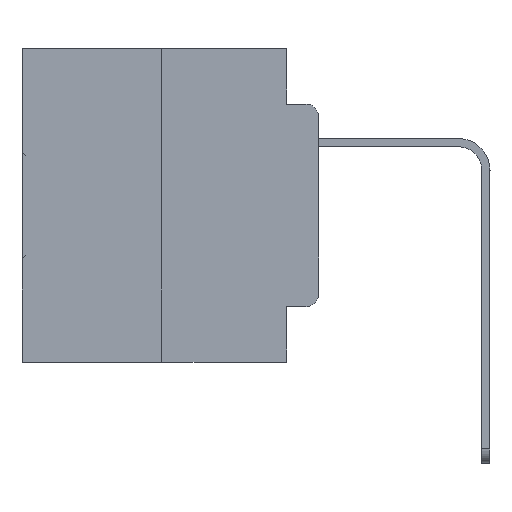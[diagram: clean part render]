
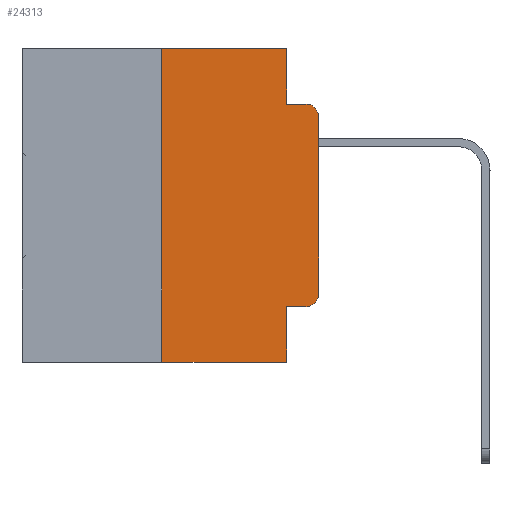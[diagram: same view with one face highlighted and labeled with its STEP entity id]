
A CAD part, left-side view. The second image highlights one B-rep face of the part: STEP entity #24313.
In plain terms, the highlighted planar face has unit normal (-1, 0, 0).
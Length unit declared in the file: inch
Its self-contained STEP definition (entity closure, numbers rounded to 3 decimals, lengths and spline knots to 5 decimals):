
#110 = VERTEX_POINT ( 'NONE', #16568 ) ;
#648 = CARTESIAN_POINT ( 'NONE',  ( 0., 0.473, 0. ) ) ;
#1026 = VERTEX_POINT ( 'NONE', #14352 ) ;
#2421 = EDGE_CURVE ( 'NONE', #32405, #26979, #25047, .T. ) ;
#2509 = ORIENTED_EDGE ( 'NONE', *, *, #9516, .F. ) ;
#2989 = CARTESIAN_POINT ( 'NONE',  ( 0., 0.051, -0.5 ) ) ;
#3905 = DIRECTION ( 'NONE',  ( 0., 0., -1. ) ) ;
#3962 = CARTESIAN_POINT ( 'NONE',  ( 0., 0.02, -0.3915 ) ) ;
#4228 = VERTEX_POINT ( 'NONE', #2989 ) ;
#4620 = VECTOR ( 'NONE', #25881, 39.37008 ) ;
#4867 = DIRECTION ( 'NONE',  ( 0., -1., 0. ) ) ;
#5163 = CARTESIAN_POINT ( 'NONE',  ( 0., 0.051, -0.0885 ) ) ;
#5921 = CARTESIAN_POINT ( 'NONE',  ( 0., 0.02, -0.4115 ) ) ;
#6248 = EDGE_CURVE ( 'NONE', #14965, #32405, #28754, .T. ) ;
#7093 = ORIENTED_EDGE ( 'NONE', *, *, #7260, .F. ) ;
#7141 = DIRECTION ( 'NONE',  ( 0., 0., 1. ) ) ;
#7260 = EDGE_CURVE ( 'NONE', #32415, #110, #22775, .T. ) ;
#7459 = VERTEX_POINT ( 'NONE', #29236 ) ;
#7633 = VERTEX_POINT ( 'NONE', #25084 ) ;
#8470 = ORIENTED_EDGE ( 'NONE', *, *, #11380, .T. ) ;
#8728 = DIRECTION ( 'NONE',  ( 0., 0., -1. ) ) ;
#8834 = VECTOR ( 'NONE', #23451, 39.37008 ) ;
#8959 = PLANE ( 'NONE',  #24630 ) ;
#9076 = VERTEX_POINT ( 'NONE', #15809 ) ;
#9467 = CARTESIAN_POINT ( 'NONE',  ( 0., 0., -0.1085 ) ) ;
#9516 = EDGE_CURVE ( 'NONE', #9076, #1026, #17217, .T. ) ;
#9683 = ORIENTED_EDGE ( 'NONE', *, *, #17641, .F. ) ;
#10777 = CARTESIAN_POINT ( 'NONE',  ( 0., 0.051, 0. ) ) ;
#11125 = ORIENTED_EDGE ( 'NONE', *, *, #31352, .F. ) ;
#11380 = EDGE_CURVE ( 'NONE', #9076, #4228, #19839, .T. ) ;
#12059 = VECTOR ( 'NONE', #20647, 39.37008 ) ;
#12429 = DIRECTION ( 'NONE',  ( 0., 0., 1. ) ) ;
#12654 = FACE_OUTER_BOUND ( 'NONE', #20829, .T. ) ;
#13606 = DIRECTION ( 'NONE',  ( -1., 0., 0. ) ) ;
#13835 = CARTESIAN_POINT ( 'NONE',  ( 0., 0.473, 0. ) ) ;
#13937 = DIRECTION ( 'NONE',  ( 0., 0., -1. ) ) ;
#14352 = CARTESIAN_POINT ( 'NONE',  ( 0., 0.25, 0. ) ) ;
#14561 = VECTOR ( 'NONE', #24209, 39.37008 ) ;
#14803 = LINE ( 'NONE', #648, #8834 ) ;
#14965 = VERTEX_POINT ( 'NONE', #5921 ) ;
#14976 = CARTESIAN_POINT ( 'NONE',  ( 0., 0.473, -0.5 ) ) ;
#15809 = CARTESIAN_POINT ( 'NONE',  ( 0., 0.25, -0.5 ) ) ;
#16126 = LINE ( 'NONE', #18739, #14561 ) ;
#16568 = CARTESIAN_POINT ( 'NONE',  ( 0., 0.02, -0.0885 ) ) ;
#17217 = LINE ( 'NONE', #19981, #27925 ) ;
#17641 = EDGE_CURVE ( 'NONE', #7633, #32415, #30354, .T. ) ;
#18279 = VECTOR ( 'NONE', #7141, 39.37008 ) ;
#18739 = CARTESIAN_POINT ( 'NONE',  ( 0., 0.051, -0.4115 ) ) ;
#18946 = ORIENTED_EDGE ( 'NONE', *, *, #19660, .F. ) ;
#19660 = EDGE_CURVE ( 'NONE', #7459, #4228, #25637, .T. ) ;
#19792 = EDGE_CURVE ( 'NONE', #7459, #14965, #16126, .T. ) ;
#19839 = LINE ( 'NONE', #14976, #20243 ) ;
#19964 = CARTESIAN_POINT ( 'NONE',  ( 0., 0., -0.3915 ) ) ;
#19981 = CARTESIAN_POINT ( 'NONE',  ( 0., 0.25, 0. ) ) ;
#20243 = VECTOR ( 'NONE', #4867, 39.37008 ) ;
#20647 = DIRECTION ( 'NONE',  ( 0., -1., 0. ) ) ;
#20829 = EDGE_LOOP ( 'NONE', ( #23954, #31686, #7093, #9683, #11125, #2509, #8470, #18946, #32541, #26570 ) ) ;
#21140 = EDGE_CURVE ( 'NONE', #26979, #110, #31125, .T. ) ;
#22475 = CARTESIAN_POINT ( 'NONE',  ( 0., 0.02, -0.1085 ) ) ;
#22626 = AXIS2_PLACEMENT_3D ( 'NONE', #22475, #32162, #27371 ) ;
#22775 = LINE ( 'NONE', #5163, #12059 ) ;
#23159 = VECTOR ( 'NONE', #3905, 39.37008 ) ;
#23451 = DIRECTION ( 'NONE',  ( 0., -1., 0. ) ) ;
#23790 = AXIS2_PLACEMENT_3D ( 'NONE', #3962, #13606, #8728 ) ;
#23954 = ORIENTED_EDGE ( 'NONE', *, *, #2421, .T. ) ;
#24209 = DIRECTION ( 'NONE',  ( 0., -1., 0. ) ) ;
#24313 = ADVANCED_FACE ( 'NONE', ( #12654 ), #8959, .F. ) ;
#24630 = AXIS2_PLACEMENT_3D ( 'NONE', #13835, #26695, #13937 ) ;
#25047 = LINE ( 'NONE', #28685, #18279 ) ;
#25084 = CARTESIAN_POINT ( 'NONE',  ( 0., 0.051, 0. ) ) ;
#25637 = LINE ( 'NONE', #10777, #4620 ) ;
#25881 = DIRECTION ( 'NONE',  ( 0., 0., -1. ) ) ;
#26570 = ORIENTED_EDGE ( 'NONE', *, *, #6248, .T. ) ;
#26695 = DIRECTION ( 'NONE',  ( 1., 0., 0. ) ) ;
#26979 = VERTEX_POINT ( 'NONE', #9467 ) ;
#27371 = DIRECTION ( 'NONE',  ( 0., 0., -1. ) ) ;
#27925 = VECTOR ( 'NONE', #12429, 39.37008 ) ;
#28685 = CARTESIAN_POINT ( 'NONE',  ( 0., 0., 0. ) ) ;
#28754 = CIRCLE ( 'NONE', #23790, 0.02 ) ;
#29092 = CARTESIAN_POINT ( 'NONE',  ( 0., 0.051, 0. ) ) ;
#29236 = CARTESIAN_POINT ( 'NONE',  ( 0., 0.051, -0.4115 ) ) ;
#30099 = CARTESIAN_POINT ( 'NONE',  ( 0., 0.051, -0.0885 ) ) ;
#30354 = LINE ( 'NONE', #29092, #23159 ) ;
#31125 = CIRCLE ( 'NONE', #22626, 0.02 ) ;
#31352 = EDGE_CURVE ( 'NONE', #1026, #7633, #14803, .T. ) ;
#31686 = ORIENTED_EDGE ( 'NONE', *, *, #21140, .T. ) ;
#32162 = DIRECTION ( 'NONE',  ( -1., 0., 0. ) ) ;
#32405 = VERTEX_POINT ( 'NONE', #19964 ) ;
#32415 = VERTEX_POINT ( 'NONE', #30099 ) ;
#32541 = ORIENTED_EDGE ( 'NONE', *, *, #19792, .T. ) ;
